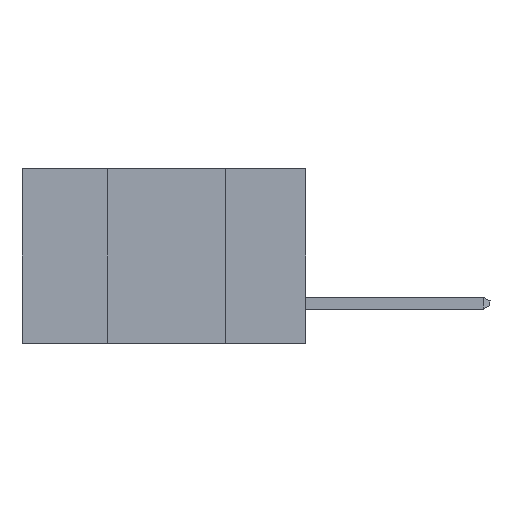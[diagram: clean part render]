
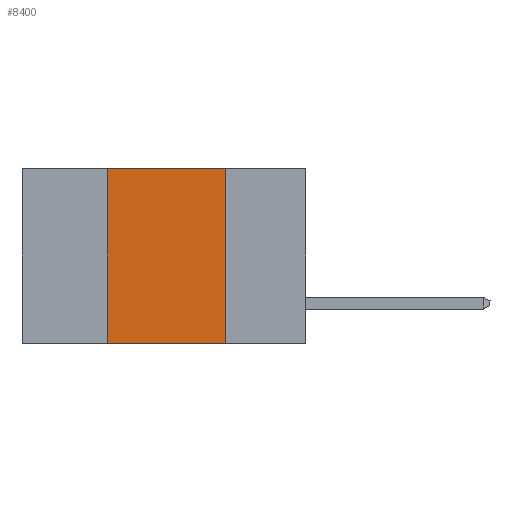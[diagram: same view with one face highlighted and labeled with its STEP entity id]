
A CAD part, left-side view. The second image highlights one B-rep face of the part: STEP entity #8400.
In plain terms, the highlighted planar face has unit normal (-1, 0, 0).
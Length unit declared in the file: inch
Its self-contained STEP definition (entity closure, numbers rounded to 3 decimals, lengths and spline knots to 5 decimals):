
#602 = VERTEX_POINT ( 'NONE', #8433 ) ;
#641 = CARTESIAN_POINT ( 'NONE',  ( 0., 0.42, 0. ) ) ;
#1437 = AXIS2_PLACEMENT_3D ( 'NONE', #8371, #3867, #4684 ) ;
#1505 = LINE ( 'NONE', #6163, #3604 ) ;
#1540 = ORIENTED_EDGE ( 'NONE', *, *, #3473, .T. ) ;
#1657 = EDGE_LOOP ( 'NONE', ( #7491, #6848, #4911, #1540 ) ) ;
#1712 = VECTOR ( 'NONE', #8596, 39.37008 ) ;
#1837 = CARTESIAN_POINT ( 'NONE',  ( 0., 0.42, -0.37 ) ) ;
#2231 = LINE ( 'NONE', #6040, #1712 ) ;
#2446 = EDGE_CURVE ( 'NONE', #6775, #602, #2231, .T. ) ;
#2518 = VECTOR ( 'NONE', #4266, 39.37008 ) ;
#3473 = EDGE_CURVE ( 'NONE', #5974, #6760, #8032, .T. ) ;
#3604 = VECTOR ( 'NONE', #9318, 39.37008 ) ;
#3867 = DIRECTION ( 'NONE',  ( 1., 0., 0. ) ) ;
#4266 = DIRECTION ( 'NONE',  ( 0., -1., 0. ) ) ;
#4336 = FACE_OUTER_BOUND ( 'NONE', #1657, .T. ) ;
#4684 = DIRECTION ( 'NONE',  ( 0., 0., -1. ) ) ;
#4793 = EDGE_CURVE ( 'NONE', #602, #6760, #8769, .T. ) ;
#4911 = ORIENTED_EDGE ( 'NONE', *, *, #9686, .F. ) ;
#5584 = CARTESIAN_POINT ( 'NONE',  ( 0., 0.6, -0.37 ) ) ;
#5974 = VERTEX_POINT ( 'NONE', #1837 ) ;
#6040 = CARTESIAN_POINT ( 'NONE',  ( 0., 0.6, 0. ) ) ;
#6163 = CARTESIAN_POINT ( 'NONE',  ( 0., 0.42, -0.37 ) ) ;
#6649 = VECTOR ( 'NONE', #7308, 39.37008 ) ;
#6760 = VERTEX_POINT ( 'NONE', #9219 ) ;
#6775 = VERTEX_POINT ( 'NONE', #641 ) ;
#6848 = ORIENTED_EDGE ( 'NONE', *, *, #2446, .F. ) ;
#7308 = DIRECTION ( 'NONE',  ( 0., 0., -1. ) ) ;
#7433 = PLANE ( 'NONE',  #1437 ) ;
#7491 = ORIENTED_EDGE ( 'NONE', *, *, #4793, .F. ) ;
#8032 = LINE ( 'NONE', #5584, #2518 ) ;
#8371 = CARTESIAN_POINT ( 'NONE',  ( 0., 0.6, 0. ) ) ;
#8400 = ADVANCED_FACE ( 'NONE', ( #4336 ), #7433, .F. ) ;
#8433 = CARTESIAN_POINT ( 'NONE',  ( 0., 0.17, 0. ) ) ;
#8596 = DIRECTION ( 'NONE',  ( 0., -1., 0. ) ) ;
#8769 = LINE ( 'NONE', #8816, #6649 ) ;
#8816 = CARTESIAN_POINT ( 'NONE',  ( 0., 0.17, -0.37 ) ) ;
#9219 = CARTESIAN_POINT ( 'NONE',  ( 0., 0.17, -0.37 ) ) ;
#9318 = DIRECTION ( 'NONE',  ( 0., 0., 1. ) ) ;
#9686 = EDGE_CURVE ( 'NONE', #5974, #6775, #1505, .T. ) ;
